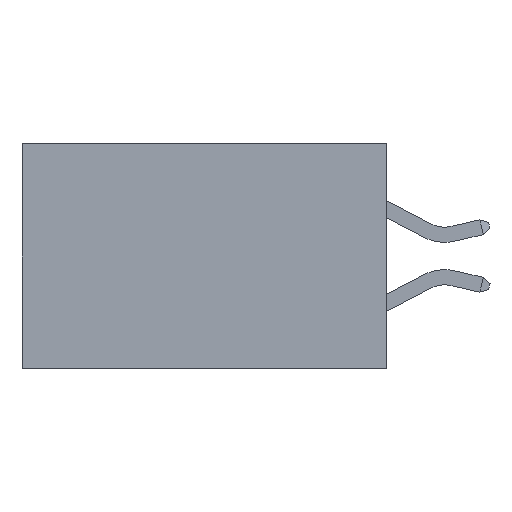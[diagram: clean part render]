
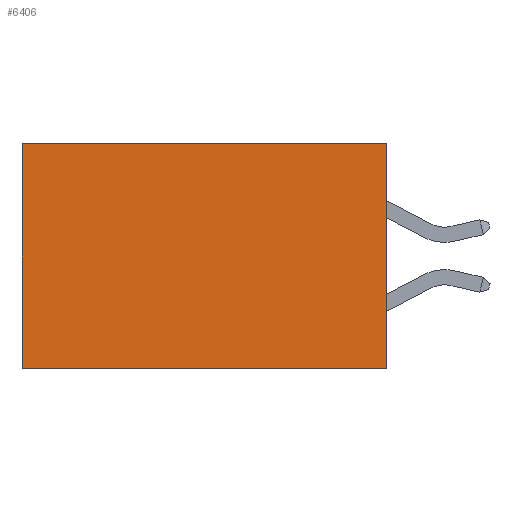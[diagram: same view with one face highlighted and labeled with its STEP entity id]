
A CAD part, left-side view. The second image highlights one B-rep face of the part: STEP entity #6406.
In plain terms, the highlighted planar face has unit normal (-1, 0, 0).
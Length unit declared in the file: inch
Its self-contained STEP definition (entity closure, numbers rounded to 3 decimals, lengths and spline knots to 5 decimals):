
#140 = ORIENTED_EDGE ( 'NONE', *, *, #20731, .T. ) ;
#882 = CARTESIAN_POINT ( 'NONE',  ( 0.2615, 0.6, 0. ) ) ;
#1549 = DIRECTION ( 'NONE',  ( 0., 1., 0. ) ) ;
#2071 = VERTEX_POINT ( 'NONE', #9264 ) ;
#2960 = VERTEX_POINT ( 'NONE', #882 ) ;
#3034 = CARTESIAN_POINT ( 'NONE',  ( 0.2615, 0., 0. ) ) ;
#6147 = EDGE_CURVE ( 'NONE', #2960, #9915, #21768, .T. ) ;
#6252 = DIRECTION ( 'NONE',  ( 0., 0., -1. ) ) ;
#6286 = DIRECTION ( 'NONE',  ( 1., 0., 0. ) ) ;
#6336 = PLANE ( 'NONE',  #24020 ) ;
#6406 = ADVANCED_FACE ( 'NONE', ( #11316 ), #6336, .F. ) ;
#6505 = CARTESIAN_POINT ( 'NONE',  ( 0.2615, 0., -0.37 ) ) ;
#7960 = VECTOR ( 'NONE', #1549, 39.37008 ) ;
#8544 = LINE ( 'NONE', #24583, #7960 ) ;
#9211 = EDGE_CURVE ( 'NONE', #14708, #2071, #24836, .T. ) ;
#9264 = CARTESIAN_POINT ( 'NONE',  ( 0.2615, 0., -0.37 ) ) ;
#9343 = DIRECTION ( 'NONE',  ( 0., 0., -1. ) ) ;
#9592 = CARTESIAN_POINT ( 'NONE',  ( 0.2615, 0.6, -0.37 ) ) ;
#9659 = LINE ( 'NONE', #20458, #24264 ) ;
#9915 = VERTEX_POINT ( 'NONE', #23779 ) ;
#10360 = CARTESIAN_POINT ( 'NONE',  ( 0.2615, 0., -0.37 ) ) ;
#10443 = DIRECTION ( 'NONE',  ( 0., 0., -1. ) ) ;
#11316 = FACE_OUTER_BOUND ( 'NONE', #24314, .T. ) ;
#11634 = VECTOR ( 'NONE', #9343, 39.37008 ) ;
#12171 = EDGE_CURVE ( 'NONE', #2071, #9915, #9659, .T. ) ;
#12245 = ORIENTED_EDGE ( 'NONE', *, *, #9211, .F. ) ;
#14708 = VERTEX_POINT ( 'NONE', #3034 ) ;
#15443 = VECTOR ( 'NONE', #10443, 39.37008 ) ;
#17195 = ORIENTED_EDGE ( 'NONE', *, *, #6147, .T. ) ;
#18548 = DIRECTION ( 'NONE',  ( 0., 1., 0. ) ) ;
#19835 = ORIENTED_EDGE ( 'NONE', *, *, #12171, .F. ) ;
#20458 = CARTESIAN_POINT ( 'NONE',  ( 0.2615, 0., -0.37 ) ) ;
#20731 = EDGE_CURVE ( 'NONE', #14708, #2960, #8544, .T. ) ;
#21768 = LINE ( 'NONE', #9592, #11634 ) ;
#23779 = CARTESIAN_POINT ( 'NONE',  ( 0.2615, 0.6, -0.37 ) ) ;
#24020 = AXIS2_PLACEMENT_3D ( 'NONE', #6505, #6286, #6252 ) ;
#24264 = VECTOR ( 'NONE', #18548, 39.37008 ) ;
#24314 = EDGE_LOOP ( 'NONE', ( #17195, #19835, #12245, #140 ) ) ;
#24583 = CARTESIAN_POINT ( 'NONE',  ( 0.2615, 0., 0. ) ) ;
#24836 = LINE ( 'NONE', #10360, #15443 ) ;
